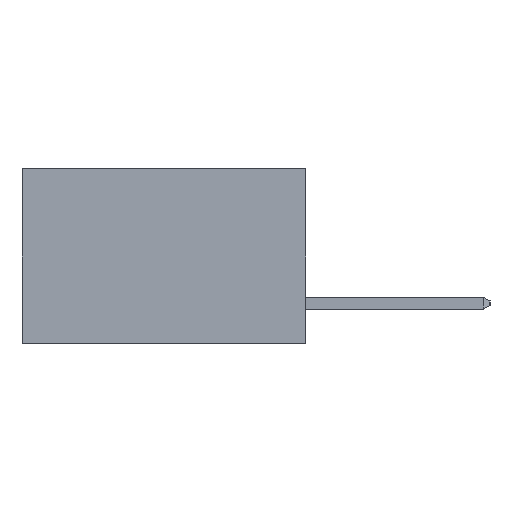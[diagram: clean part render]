
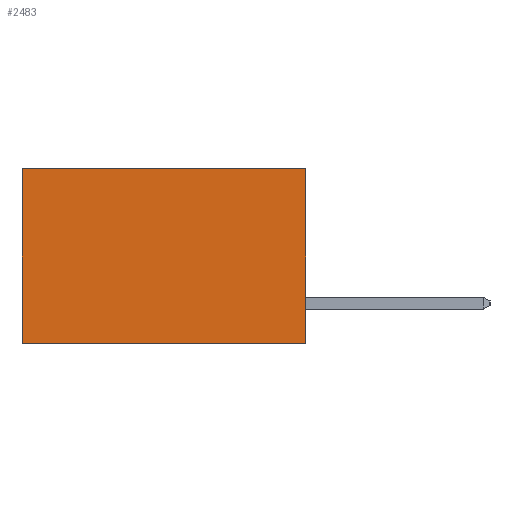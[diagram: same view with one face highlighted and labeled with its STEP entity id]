
A CAD part, left-side view. The second image highlights one B-rep face of the part: STEP entity #2483.
In plain terms, the highlighted planar face has unit normal (-1, 0, 0).
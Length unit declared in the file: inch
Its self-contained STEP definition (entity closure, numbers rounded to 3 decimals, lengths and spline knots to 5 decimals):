
#146 = VECTOR ( 'NONE', #15359, 39.37008 ) ;
#350 = EDGE_CURVE ( 'NONE', #1627, #16193, #9288, .T. ) ;
#420 = EDGE_CURVE ( 'NONE', #11716, #1627, #13906, .T. ) ;
#603 = ORIENTED_EDGE ( 'NONE', *, *, #350, .F. ) ;
#769 = ORIENTED_EDGE ( 'NONE', *, *, #420, .F. ) ;
#1627 = VERTEX_POINT ( 'NONE', #4369 ) ;
#1816 = EDGE_CURVE ( 'NONE', #8334, #16193, #7424, .T. ) ;
#1974 = ORIENTED_EDGE ( 'NONE', *, *, #11393, .T. ) ;
#2286 = VECTOR ( 'NONE', #9045, 39.37008 ) ;
#2483 = ADVANCED_FACE ( 'NONE', ( #6019 ), #6151, .F. ) ;
#2829 = DIRECTION ( 'NONE',  ( 0., 1., 0. ) ) ;
#3539 = DIRECTION ( 'NONE',  ( 0., 0., -1. ) ) ;
#3910 = ORIENTED_EDGE ( 'NONE', *, *, #1816, .T. ) ;
#4369 = CARTESIAN_POINT ( 'NONE',  ( 0.2615, 0., -0.37 ) ) ;
#4497 = DIRECTION ( 'NONE',  ( 1., 0., 0. ) ) ;
#5880 = CARTESIAN_POINT ( 'NONE',  ( 0.2615, 0., -0.37 ) ) ;
#5895 = CARTESIAN_POINT ( 'NONE',  ( 0.2615, 0., -0.37 ) ) ;
#6019 = FACE_OUTER_BOUND ( 'NONE', #15606, .T. ) ;
#6151 = PLANE ( 'NONE',  #6254 ) ;
#6254 = AXIS2_PLACEMENT_3D ( 'NONE', #5895, #4497, #3539 ) ;
#6763 = LINE ( 'NONE', #16733, #16269 ) ;
#7424 = LINE ( 'NONE', #13203, #146 ) ;
#7569 = CARTESIAN_POINT ( 'NONE',  ( 0.2615, 0., -0.37 ) ) ;
#8334 = VERTEX_POINT ( 'NONE', #11815 ) ;
#9045 = DIRECTION ( 'NONE',  ( 0., 1., 0. ) ) ;
#9288 = LINE ( 'NONE', #7569, #2286 ) ;
#10203 = CARTESIAN_POINT ( 'NONE',  ( 0.2615, 0., 0. ) ) ;
#10660 = VECTOR ( 'NONE', #12741, 39.37008 ) ;
#10831 = CARTESIAN_POINT ( 'NONE',  ( 0.2615, 0.6, -0.37 ) ) ;
#11393 = EDGE_CURVE ( 'NONE', #11716, #8334, #6763, .T. ) ;
#11716 = VERTEX_POINT ( 'NONE', #10203 ) ;
#11815 = CARTESIAN_POINT ( 'NONE',  ( 0.2615, 0.6, 0. ) ) ;
#12741 = DIRECTION ( 'NONE',  ( 0., 0., -1. ) ) ;
#13203 = CARTESIAN_POINT ( 'NONE',  ( 0.2615, 0.6, -0.37 ) ) ;
#13906 = LINE ( 'NONE', #5880, #10660 ) ;
#15359 = DIRECTION ( 'NONE',  ( 0., 0., -1. ) ) ;
#15606 = EDGE_LOOP ( 'NONE', ( #3910, #603, #769, #1974 ) ) ;
#16193 = VERTEX_POINT ( 'NONE', #10831 ) ;
#16269 = VECTOR ( 'NONE', #2829, 39.37008 ) ;
#16733 = CARTESIAN_POINT ( 'NONE',  ( 0.2615, 0., 0. ) ) ;
